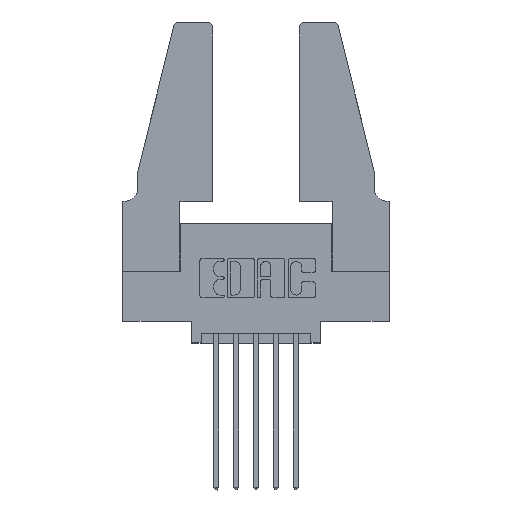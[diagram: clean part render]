
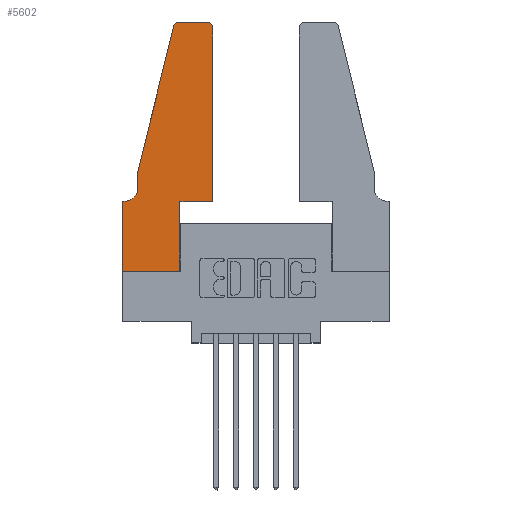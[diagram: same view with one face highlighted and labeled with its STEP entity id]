
A CAD part, top view. The second image highlights one B-rep face of the part: STEP entity #5602.
In plain terms, the highlighted planar face has unit normal (0, 0, 1).
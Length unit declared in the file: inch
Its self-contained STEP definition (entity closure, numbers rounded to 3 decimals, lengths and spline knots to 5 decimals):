
#56 = VECTOR ( 'NONE', #8714, 39.37008 ) ;
#65 = EDGE_CURVE ( 'NONE', #8882, #4059, #832, .T. ) ;
#136 = CARTESIAN_POINT ( 'NONE',  ( 0.0055, 0.42, 0.37 ) ) ;
#317 = LINE ( 'NONE', #1353, #1543 ) ;
#332 = CARTESIAN_POINT ( 'NONE',  ( 0.4205, 1.25, 0.37 ) ) ;
#339 = DIRECTION ( 'NONE',  ( 0., 0., 1. ) ) ;
#370 = ORIENTED_EDGE ( 'NONE', *, *, #5862, .T. ) ;
#415 = VERTEX_POINT ( 'NONE', #1814 ) ;
#524 = DIRECTION ( 'NONE',  ( 0., -1., 0. ) ) ;
#570 = VECTOR ( 'NONE', #5708, 39.37008 ) ;
#606 = VERTEX_POINT ( 'NONE', #332 ) ;
#616 = DIRECTION ( 'NONE',  ( 0., 1., 0. ) ) ;
#832 = LINE ( 'NONE', #8932, #6001 ) ;
#957 = PLANE ( 'NONE',  #3260 ) ;
#1025 = DIRECTION ( 'NONE',  ( 0., 0., -1. ) ) ;
#1353 = CARTESIAN_POINT ( 'NONE',  ( 0.2865, 0.35, 0.37 ) ) ;
#1495 = VERTEX_POINT ( 'NONE', #6456 ) ;
#1503 = VECTOR ( 'NONE', #524, 39.37008 ) ;
#1543 = VECTOR ( 'NONE', #616, 39.37008 ) ;
#1601 = CARTESIAN_POINT ( 'NONE',  ( 0.4505, 0.35, 0.37 ) ) ;
#1713 = DIRECTION ( 'NONE',  ( -1., 0., 0. ) ) ;
#1814 = CARTESIAN_POINT ( 'NONE',  ( 0.4505, 1.22, 0.37 ) ) ;
#2098 = DIRECTION ( 'NONE',  ( 1., 0., 0. ) ) ;
#2126 = ORIENTED_EDGE ( 'NONE', *, *, #8054, .T. ) ;
#2324 = VECTOR ( 'NONE', #9670, 39.37008 ) ;
#2612 = ORIENTED_EDGE ( 'NONE', *, *, #3614, .T. ) ;
#2755 = AXIS2_PLACEMENT_3D ( 'NONE', #5523, #339, #2098 ) ;
#2812 = DIRECTION ( 'NONE',  ( -1., 0., 0. ) ) ;
#3061 = ORIENTED_EDGE ( 'NONE', *, *, #5110, .T. ) ;
#3094 = ORIENTED_EDGE ( 'NONE', *, *, #65, .T. ) ;
#3260 = AXIS2_PLACEMENT_3D ( 'NONE', #7842, #7103, #3568 ) ;
#3432 = VERTEX_POINT ( 'NONE', #4870 ) ;
#3453 = CIRCLE ( 'NONE', #6231, 0.07 ) ;
#3477 = CARTESIAN_POINT ( 'NONE',  ( 0.4505, 0.35, 0.37 ) ) ;
#3503 = ORIENTED_EDGE ( 'NONE', *, *, #5618, .T. ) ;
#3568 = DIRECTION ( 'NONE',  ( 1., 0., 0. ) ) ;
#3614 = EDGE_CURVE ( 'NONE', #3432, #1495, #8325, .T. ) ;
#3762 = CARTESIAN_POINT ( 'NONE',  ( 0.0755, 0.35, 0.37 ) ) ;
#3974 = VERTEX_POINT ( 'NONE', #4583 ) ;
#4059 = VERTEX_POINT ( 'NONE', #11011 ) ;
#4283 = EDGE_CURVE ( 'NONE', #3974, #3432, #317, .T. ) ;
#4490 = VERTEX_POINT ( 'NONE', #8446 ) ;
#4583 = CARTESIAN_POINT ( 'NONE',  ( 0.2865, 0., 0.37 ) ) ;
#4654 = VECTOR ( 'NONE', #4683, 39.37008 ) ;
#4683 = DIRECTION ( 'NONE',  ( -1., 0., 0. ) ) ;
#4796 = VECTOR ( 'NONE', #5034, 39.37008 ) ;
#4870 = CARTESIAN_POINT ( 'NONE',  ( 0.2865, 0.35, 0.37 ) ) ;
#4979 = CARTESIAN_POINT ( 'NONE',  ( 0.284, 1.22, 0.37 ) ) ;
#4986 = CARTESIAN_POINT ( 'NONE',  ( 0.0755, 0.5, 0.37 ) ) ;
#5034 = DIRECTION ( 'NONE',  ( 0., 1., 0. ) ) ;
#5072 = ORIENTED_EDGE ( 'NONE', *, *, #7804, .T. ) ;
#5110 = EDGE_CURVE ( 'NONE', #1495, #415, #8566, .T. ) ;
#5201 = EDGE_CURVE ( 'NONE', #10067, #4490, #3453, .T. ) ;
#5208 = EDGE_LOOP ( 'NONE', ( #5072, #2126, #370, #9893, #6206, #7920, #3094, #3503, #10115, #2612, #3061, #10774 ) ) ;
#5317 = VERTEX_POINT ( 'NONE', #5575 ) ;
#5523 = CARTESIAN_POINT ( 'NONE',  ( 0.4205, 1.22, 0.37 ) ) ;
#5575 = CARTESIAN_POINT ( 'NONE',  ( 0.284, 1.25, 0.37 ) ) ;
#5602 = ADVANCED_FACE ( 'NONE', ( #6417 ), #957, .T. ) ;
#5618 = EDGE_CURVE ( 'NONE', #4059, #3974, #7092, .T. ) ;
#5708 = DIRECTION ( 'NONE',  ( -0.239, -0.971, 0. ) ) ;
#5734 = LINE ( 'NONE', #3762, #4654 ) ;
#5862 = EDGE_CURVE ( 'NONE', #9072, #8896, #10467, .T. ) ;
#5881 = DIRECTION ( 'NONE',  ( 1., 0., 0. ) ) ;
#5913 = CARTESIAN_POINT ( 'NONE',  ( 0.25487, 1.22718, 0.37 ) ) ;
#6001 = VECTOR ( 'NONE', #7056, 39.37008 ) ;
#6206 = ORIENTED_EDGE ( 'NONE', *, *, #5201, .T. ) ;
#6210 = CARTESIAN_POINT ( 'NONE',  ( 0., 0., 0.37 ) ) ;
#6231 = AXIS2_PLACEMENT_3D ( 'NONE', #136, #1025, #2812 ) ;
#6409 = EDGE_CURVE ( 'NONE', #4490, #8882, #5734, .T. ) ;
#6416 = VECTOR ( 'NONE', #1713, 39.37008 ) ;
#6417 = FACE_OUTER_BOUND ( 'NONE', #5208, .T. ) ;
#6456 = CARTESIAN_POINT ( 'NONE',  ( 0.4505, 0.35, 0.37 ) ) ;
#6596 = AXIS2_PLACEMENT_3D ( 'NONE', #4979, #11001, #5881 ) ;
#6961 = EDGE_CURVE ( 'NONE', #8896, #10067, #11108, .T. ) ;
#7056 = DIRECTION ( 'NONE',  ( 0., -1., 0. ) ) ;
#7092 = LINE ( 'NONE', #6210, #2324 ) ;
#7103 = DIRECTION ( 'NONE',  ( 0., 0., 1. ) ) ;
#7426 = EDGE_CURVE ( 'NONE', #415, #606, #8700, .T. ) ;
#7716 = CARTESIAN_POINT ( 'NONE',  ( 0.2605, 1.25, 0.37 ) ) ;
#7804 = EDGE_CURVE ( 'NONE', #606, #5317, #8012, .T. ) ;
#7842 = CARTESIAN_POINT ( 'NONE',  ( 0., 0.35, 0.37 ) ) ;
#7920 = ORIENTED_EDGE ( 'NONE', *, *, #6409, .T. ) ;
#7924 = CARTESIAN_POINT ( 'NONE',  ( 0.0755, 0.42, 0.37 ) ) ;
#8012 = LINE ( 'NONE', #7716, #6416 ) ;
#8054 = EDGE_CURVE ( 'NONE', #5317, #9072, #8821, .T. ) ;
#8325 = LINE ( 'NONE', #3477, #56 ) ;
#8446 = CARTESIAN_POINT ( 'NONE',  ( 0.0055, 0.35, 0.37 ) ) ;
#8566 = LINE ( 'NONE', #1601, #4796 ) ;
#8700 = CIRCLE ( 'NONE', #2755, 0.03 ) ;
#8714 = DIRECTION ( 'NONE',  ( 1., 0., 0. ) ) ;
#8821 = CIRCLE ( 'NONE', #6596, 0.03 ) ;
#8882 = VERTEX_POINT ( 'NONE', #9280 ) ;
#8896 = VERTEX_POINT ( 'NONE', #9521 ) ;
#8932 = CARTESIAN_POINT ( 'NONE',  ( 0., 0., 0.37 ) ) ;
#9072 = VERTEX_POINT ( 'NONE', #5913 ) ;
#9280 = CARTESIAN_POINT ( 'NONE',  ( 0., 0.35, 0.37 ) ) ;
#9521 = CARTESIAN_POINT ( 'NONE',  ( 0.0755, 0.5, 0.37 ) ) ;
#9670 = DIRECTION ( 'NONE',  ( 1., 0., 0. ) ) ;
#9893 = ORIENTED_EDGE ( 'NONE', *, *, #6961, .T. ) ;
#10067 = VERTEX_POINT ( 'NONE', #7924 ) ;
#10115 = ORIENTED_EDGE ( 'NONE', *, *, #4283, .T. ) ;
#10467 = LINE ( 'NONE', #11017, #570 ) ;
#10774 = ORIENTED_EDGE ( 'NONE', *, *, #7426, .T. ) ;
#11001 = DIRECTION ( 'NONE',  ( 0., 0., 1. ) ) ;
#11011 = CARTESIAN_POINT ( 'NONE',  ( 0., 0., 0.37 ) ) ;
#11017 = CARTESIAN_POINT ( 'NONE',  ( 0.0755, 0.5, 0.37 ) ) ;
#11108 = LINE ( 'NONE', #4986, #1503 ) ;
